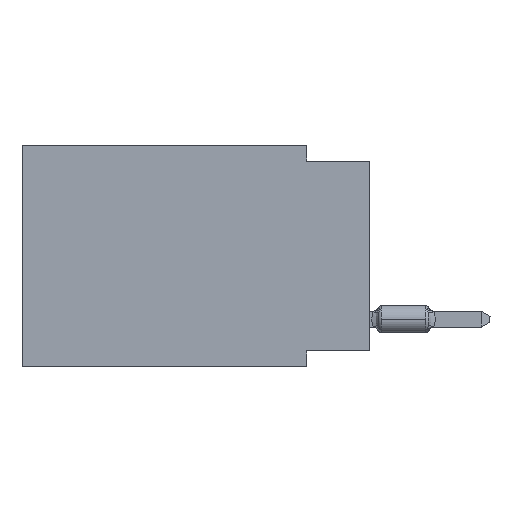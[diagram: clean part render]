
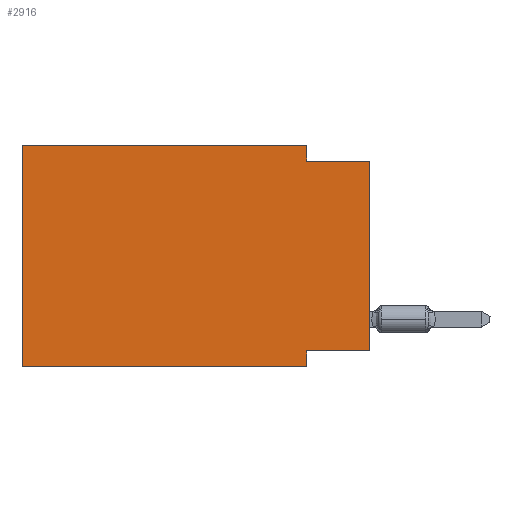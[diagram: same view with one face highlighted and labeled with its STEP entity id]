
A CAD part, left-side view. The second image highlights one B-rep face of the part: STEP entity #2916.
In plain terms, the highlighted planar face has unit normal (-1, 0, 0).
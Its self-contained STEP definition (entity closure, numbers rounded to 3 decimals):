
#2367 = LINE ( 'NONE', #47739, #9880 ) ;
#2487 = ORIENTED_EDGE ( 'NONE', *, *, #28180, .F. ) ;
#2916 = ADVANCED_FACE ( 'NONE', ( #17639 ), #3207, .F. ) ;
#3207 = PLANE ( 'NONE',  #43707 ) ;
#3535 = CARTESIAN_POINT ( 'NONE',  ( 0., 2.54, 0. ) ) ;
#4848 = VERTEX_POINT ( 'NONE', #7124 ) ;
#5372 = LINE ( 'NONE', #36893, #52477 ) ;
#7124 = CARTESIAN_POINT ( 'NONE',  ( 0., 13.97, 0. ) ) ;
#7292 = ORIENTED_EDGE ( 'NONE', *, *, #21552, .F. ) ;
#8374 = DIRECTION ( 'NONE',  ( 0., 0., -1. ) ) ;
#8912 = CARTESIAN_POINT ( 'NONE',  ( 0., 2.54, -8.255 ) ) ;
#9278 = VECTOR ( 'NONE', #9593, 1000. ) ;
#9548 = VERTEX_POINT ( 'NONE', #14566 ) ;
#9593 = DIRECTION ( 'NONE',  ( 0., -1., 0. ) ) ;
#9880 = VECTOR ( 'NONE', #38782, 1000. ) ;
#10061 = DIRECTION ( 'NONE',  ( 0., -1., 0. ) ) ;
#10311 = VERTEX_POINT ( 'NONE', #12579 ) ;
#10892 = ORIENTED_EDGE ( 'NONE', *, *, #24483, .F. ) ;
#12433 = CARTESIAN_POINT ( 'NONE',  ( 0., 13.97, 0. ) ) ;
#12579 = CARTESIAN_POINT ( 'NONE',  ( 0., 0., -0.635 ) ) ;
#14025 = VERTEX_POINT ( 'NONE', #41512 ) ;
#14566 = CARTESIAN_POINT ( 'NONE',  ( 0., 0., -8.255 ) ) ;
#14681 = CARTESIAN_POINT ( 'NONE',  ( 0., 13.97, -8.89 ) ) ;
#14842 = ORIENTED_EDGE ( 'NONE', *, *, #23964, .F. ) ;
#16003 = VERTEX_POINT ( 'NONE', #25774 ) ;
#17416 = ORIENTED_EDGE ( 'NONE', *, *, #18872, .T. ) ;
#17639 = FACE_OUTER_BOUND ( 'NONE', #39753, .T. ) ;
#18742 = LINE ( 'NONE', #14681, #33657 ) ;
#18872 = EDGE_CURVE ( 'NONE', #9548, #10311, #37894, .T. ) ;
#20018 = LINE ( 'NONE', #20298, #45918 ) ;
#20241 = VERTEX_POINT ( 'NONE', #3535 ) ;
#20298 = CARTESIAN_POINT ( 'NONE',  ( 0., 2.54, -8.89 ) ) ;
#20575 = ORIENTED_EDGE ( 'NONE', *, *, #34938, .T. ) ;
#21552 = EDGE_CURVE ( 'NONE', #45533, #10311, #35930, .T. ) ;
#23964 = EDGE_CURVE ( 'NONE', #4848, #20241, #5372, .T. ) ;
#24483 = EDGE_CURVE ( 'NONE', #26713, #14025, #20018, .T. ) ;
#25774 = CARTESIAN_POINT ( 'NONE',  ( 0., 13.97, -8.89 ) ) ;
#26086 = EDGE_CURVE ( 'NONE', #16003, #4848, #2367, .T. ) ;
#26713 = VERTEX_POINT ( 'NONE', #8912 ) ;
#27600 = ORIENTED_EDGE ( 'NONE', *, *, #26086, .F. ) ;
#28180 = EDGE_CURVE ( 'NONE', #20241, #45533, #43004, .T. ) ;
#29698 = DIRECTION ( 'NONE',  ( 0., 0., -1. ) ) ;
#30065 = DIRECTION ( 'NONE',  ( 0., 0., 1. ) ) ;
#32848 = ORIENTED_EDGE ( 'NONE', *, *, #35140, .F. ) ;
#33657 = VECTOR ( 'NONE', #10061, 1000. ) ;
#33844 = CARTESIAN_POINT ( 'NONE',  ( 0., 0., 0. ) ) ;
#34145 = DIRECTION ( 'NONE',  ( 1., 0., 0. ) ) ;
#34938 = EDGE_CURVE ( 'NONE', #16003, #14025, #18742, .T. ) ;
#35140 = EDGE_CURVE ( 'NONE', #9548, #26713, #38642, .T. ) ;
#35930 = LINE ( 'NONE', #53580, #9278 ) ;
#36893 = CARTESIAN_POINT ( 'NONE',  ( 0., 13.97, 0. ) ) ;
#37894 = LINE ( 'NONE', #33844, #46927 ) ;
#38284 = VECTOR ( 'NONE', #55448, 1000. ) ;
#38642 = LINE ( 'NONE', #51669, #38284 ) ;
#38782 = DIRECTION ( 'NONE',  ( 0., 0., 1. ) ) ;
#39451 = VECTOR ( 'NONE', #29698, 1000. ) ;
#39753 = EDGE_LOOP ( 'NONE', ( #17416, #7292, #2487, #14842, #27600, #20575, #10892, #32848 ) ) ;
#41512 = CARTESIAN_POINT ( 'NONE',  ( 0., 2.54, -8.89 ) ) ;
#43004 = LINE ( 'NONE', #47613, #39451 ) ;
#43707 = AXIS2_PLACEMENT_3D ( 'NONE', #12433, #34145, #8374 ) ;
#45533 = VERTEX_POINT ( 'NONE', #45597 ) ;
#45597 = CARTESIAN_POINT ( 'NONE',  ( 0., 2.54, -0.635 ) ) ;
#45918 = VECTOR ( 'NONE', #46331, 1000. ) ;
#46331 = DIRECTION ( 'NONE',  ( 0., 0., -1. ) ) ;
#46927 = VECTOR ( 'NONE', #30065, 1000. ) ;
#47613 = CARTESIAN_POINT ( 'NONE',  ( 0., 2.54, 0. ) ) ;
#47739 = CARTESIAN_POINT ( 'NONE',  ( 0., 13.97, 0. ) ) ;
#49618 = DIRECTION ( 'NONE',  ( 0., -1., 0. ) ) ;
#51669 = CARTESIAN_POINT ( 'NONE',  ( 0., 0., -8.255 ) ) ;
#52477 = VECTOR ( 'NONE', #49618, 1000. ) ;
#53580 = CARTESIAN_POINT ( 'NONE',  ( 0., 0., -0.635 ) ) ;
#55448 = DIRECTION ( 'NONE',  ( 0., 1., 0. ) ) ;
